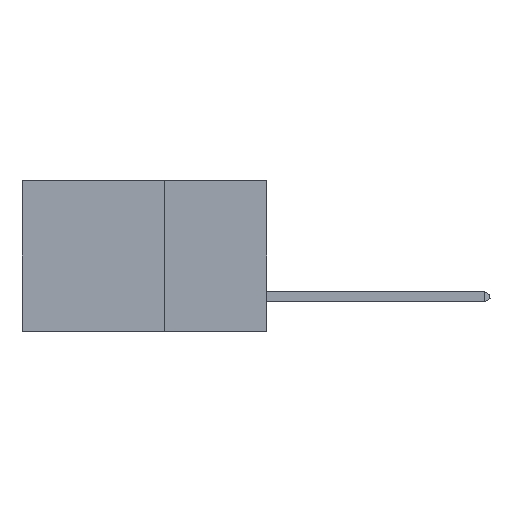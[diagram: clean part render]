
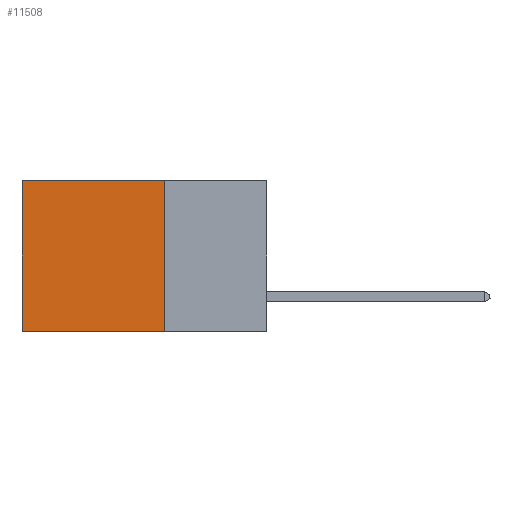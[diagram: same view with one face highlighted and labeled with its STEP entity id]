
A CAD part, left-side view. The second image highlights one B-rep face of the part: STEP entity #11508.
In plain terms, the highlighted planar face has unit normal (-1, 0, 0).
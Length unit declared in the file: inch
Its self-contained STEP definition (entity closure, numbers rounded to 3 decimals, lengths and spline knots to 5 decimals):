
#2811 = VERTEX_POINT ( 'NONE', #7646 ) ;
#3056 = VECTOR ( 'NONE', #3560, 39.37008 ) ;
#3276 = CARTESIAN_POINT ( 'NONE',  ( 0.2875, 0.25, 0. ) ) ;
#3279 = AXIS2_PLACEMENT_3D ( 'NONE', #17331, #24113, #10651 ) ;
#3407 = VERTEX_POINT ( 'NONE', #3906 ) ;
#3560 = DIRECTION ( 'NONE',  ( 0., 0., -1. ) ) ;
#3906 = CARTESIAN_POINT ( 'NONE',  ( 0.2875, 0.25, -0.37 ) ) ;
#4258 = EDGE_CURVE ( 'NONE', #3407, #26590, #11285, .T. ) ;
#4444 = DIRECTION ( 'NONE',  ( 0., 1., 0. ) ) ;
#5221 = ORIENTED_EDGE ( 'NONE', *, *, #25173, .T. ) ;
#5453 = VECTOR ( 'NONE', #16743, 39.37008 ) ;
#5599 = EDGE_LOOP ( 'NONE', ( #12150, #15882, #5768, #5221 ) ) ;
#5657 = EDGE_CURVE ( 'NONE', #29077, #26590, #8707, .T. ) ;
#5768 = ORIENTED_EDGE ( 'NONE', *, *, #22513, .F. ) ;
#7646 = CARTESIAN_POINT ( 'NONE',  ( 0.2875, 0.25, 0. ) ) ;
#8140 = FACE_OUTER_BOUND ( 'NONE', #5599, .T. ) ;
#8707 = LINE ( 'NONE', #17226, #3056 ) ;
#10651 = DIRECTION ( 'NONE',  ( 0., 0., -1. ) ) ;
#11285 = LINE ( 'NONE', #23434, #21489 ) ;
#11508 = ADVANCED_FACE ( 'NONE', ( #8140 ), #12823, .F. ) ;
#12150 = ORIENTED_EDGE ( 'NONE', *, *, #5657, .T. ) ;
#12823 = PLANE ( 'NONE',  #3279 ) ;
#13436 = LINE ( 'NONE', #24781, #25727 ) ;
#15171 = CARTESIAN_POINT ( 'NONE',  ( 0.2875, 0.6, 0. ) ) ;
#15882 = ORIENTED_EDGE ( 'NONE', *, *, #4258, .F. ) ;
#16743 = DIRECTION ( 'NONE',  ( 0., 0., -1. ) ) ;
#17226 = CARTESIAN_POINT ( 'NONE',  ( 0.2875, 0.6, 0. ) ) ;
#17331 = CARTESIAN_POINT ( 'NONE',  ( 0.2875, 0.25, 0. ) ) ;
#17428 = LINE ( 'NONE', #3276, #5453 ) ;
#17894 = CARTESIAN_POINT ( 'NONE',  ( 0.2875, 0.6, -0.37 ) ) ;
#21489 = VECTOR ( 'NONE', #25686, 39.37008 ) ;
#22513 = EDGE_CURVE ( 'NONE', #2811, #3407, #17428, .T. ) ;
#23434 = CARTESIAN_POINT ( 'NONE',  ( 0.2875, 0.25, -0.37 ) ) ;
#24113 = DIRECTION ( 'NONE',  ( 1., 0., 0. ) ) ;
#24781 = CARTESIAN_POINT ( 'NONE',  ( 0.2875, 0.25, 0. ) ) ;
#25173 = EDGE_CURVE ( 'NONE', #2811, #29077, #13436, .T. ) ;
#25686 = DIRECTION ( 'NONE',  ( 0., 1., 0. ) ) ;
#25727 = VECTOR ( 'NONE', #4444, 39.37008 ) ;
#26590 = VERTEX_POINT ( 'NONE', #17894 ) ;
#29077 = VERTEX_POINT ( 'NONE', #15171 ) ;
